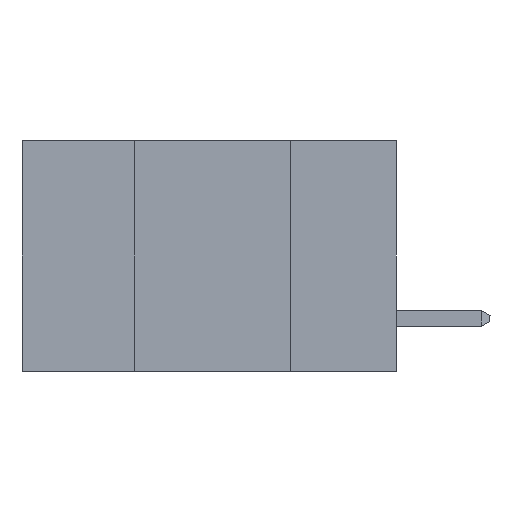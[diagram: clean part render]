
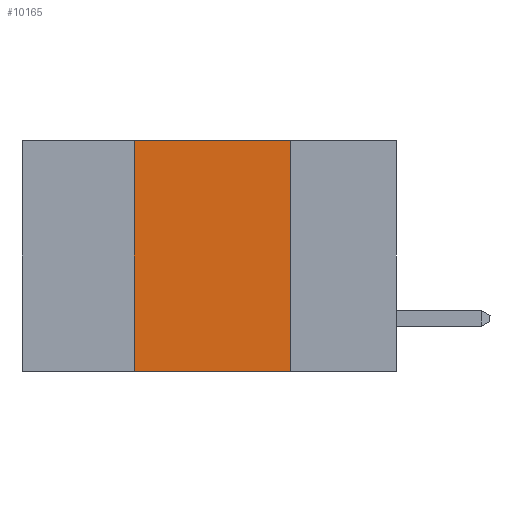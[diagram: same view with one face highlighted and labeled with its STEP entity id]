
A CAD part, left-side view. The second image highlights one B-rep face of the part: STEP entity #10165.
In plain terms, the highlighted planar face has unit normal (-1, 0, 0).
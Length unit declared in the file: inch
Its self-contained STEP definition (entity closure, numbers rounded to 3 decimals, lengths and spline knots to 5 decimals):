
#300 = VERTEX_POINT ( 'NONE', #5357 ) ;
#519 = ORIENTED_EDGE ( 'NONE', *, *, #5044, .F. ) ;
#645 = EDGE_CURVE ( 'NONE', #1228, #6062, #7066, .T. ) ;
#853 = DIRECTION ( 'NONE',  ( 0., 0., -1. ) ) ;
#1114 = VECTOR ( 'NONE', #1887, 39.37008 ) ;
#1154 = DIRECTION ( 'NONE',  ( 0., 0., -1. ) ) ;
#1228 = VERTEX_POINT ( 'NONE', #6472 ) ;
#1299 = VECTOR ( 'NONE', #853, 39.37008 ) ;
#1887 = DIRECTION ( 'NONE',  ( 0., -1., 0. ) ) ;
#1984 = ORIENTED_EDGE ( 'NONE', *, *, #645, .F. ) ;
#2856 = ORIENTED_EDGE ( 'NONE', *, *, #5690, .T. ) ;
#3572 = DIRECTION ( 'NONE',  ( 1., 0., 0. ) ) ;
#3797 = EDGE_CURVE ( 'NONE', #6062, #6005, #8610, .T. ) ;
#4214 = CARTESIAN_POINT ( 'NONE',  ( 0., 0.6, -0.37 ) ) ;
#5002 = LINE ( 'NONE', #4214, #1114 ) ;
#5044 = EDGE_CURVE ( 'NONE', #6005, #300, #8867, .T. ) ;
#5143 = CARTESIAN_POINT ( 'NONE',  ( 0., 0.6, 0. ) ) ;
#5240 = CARTESIAN_POINT ( 'NONE',  ( 0., 0.42, 0. ) ) ;
#5357 = CARTESIAN_POINT ( 'NONE',  ( 0., 0.17, -0.37 ) ) ;
#5388 = CARTESIAN_POINT ( 'NONE',  ( 0., 0.42, -0.37 ) ) ;
#5390 = CARTESIAN_POINT ( 'NONE',  ( 0., 0.6, 0. ) ) ;
#5690 = EDGE_CURVE ( 'NONE', #1228, #300, #5002, .T. ) ;
#5764 = CARTESIAN_POINT ( 'NONE',  ( 0., 0.17, 0. ) ) ;
#6005 = VERTEX_POINT ( 'NONE', #5764 ) ;
#6062 = VERTEX_POINT ( 'NONE', #5240 ) ;
#6145 = ORIENTED_EDGE ( 'NONE', *, *, #3797, .F. ) ;
#6198 = VECTOR ( 'NONE', #7808, 39.37008 ) ;
#6472 = CARTESIAN_POINT ( 'NONE',  ( 0., 0.42, -0.37 ) ) ;
#6969 = DIRECTION ( 'NONE',  ( 0., -1., 0. ) ) ;
#6992 = VECTOR ( 'NONE', #6969, 39.37008 ) ;
#7066 = LINE ( 'NONE', #5388, #6198 ) ;
#7808 = DIRECTION ( 'NONE',  ( 0., 0., 1. ) ) ;
#8610 = LINE ( 'NONE', #5390, #6992 ) ;
#8749 = AXIS2_PLACEMENT_3D ( 'NONE', #5143, #3572, #1154 ) ;
#8867 = LINE ( 'NONE', #10388, #1299 ) ;
#9052 = FACE_OUTER_BOUND ( 'NONE', #9069, .T. ) ;
#9069 = EDGE_LOOP ( 'NONE', ( #519, #6145, #1984, #2856 ) ) ;
#9890 = PLANE ( 'NONE',  #8749 ) ;
#10165 = ADVANCED_FACE ( 'NONE', ( #9052 ), #9890, .F. ) ;
#10388 = CARTESIAN_POINT ( 'NONE',  ( 0., 0.17, -0.37 ) ) ;
